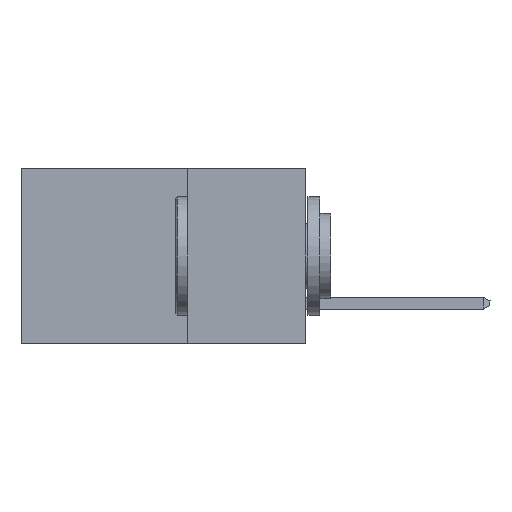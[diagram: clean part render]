
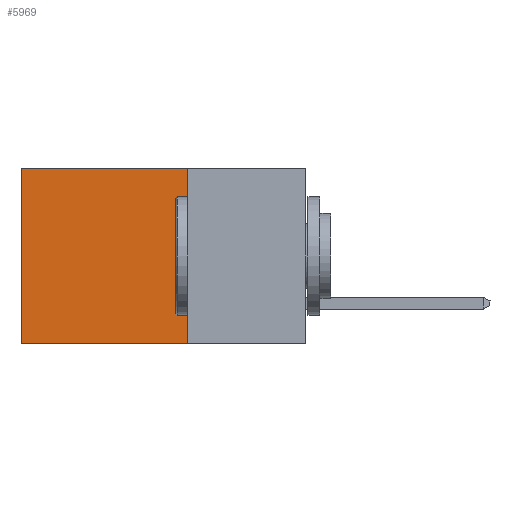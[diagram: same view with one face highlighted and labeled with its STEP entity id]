
A CAD part, left-side view. The second image highlights one B-rep face of the part: STEP entity #5969.
In plain terms, the highlighted planar face has unit normal (-1, 0, 0).
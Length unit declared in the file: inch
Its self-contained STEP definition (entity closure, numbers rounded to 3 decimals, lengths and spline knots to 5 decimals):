
#207 = VECTOR ( 'NONE', #5321, 39.37008 ) ;
#509 = EDGE_CURVE ( 'NONE', #4451, #18247, #7061, .T. ) ;
#1037 = VERTEX_POINT ( 'NONE', #16561 ) ;
#1584 = DIRECTION ( 'NONE',  ( 1., 0., 0. ) ) ;
#1895 = ORIENTED_EDGE ( 'NONE', *, *, #2058, .F. ) ;
#2058 = EDGE_CURVE ( 'NONE', #18247, #3424, #7263, .T. ) ;
#2236 = EDGE_CURVE ( 'NONE', #4451, #1037, #17257, .T. ) ;
#2767 = CARTESIAN_POINT ( 'NONE',  ( 0.298, 0.25, -0.37 ) ) ;
#2839 = VECTOR ( 'NONE', #12417, 39.37008 ) ;
#3405 = EDGE_LOOP ( 'NONE', ( #4843, #1895, #19400, #10245 ) ) ;
#3424 = VERTEX_POINT ( 'NONE', #19030 ) ;
#4451 = VERTEX_POINT ( 'NONE', #9928 ) ;
#4843 = ORIENTED_EDGE ( 'NONE', *, *, #10062, .T. ) ;
#5302 = VECTOR ( 'NONE', #11114, 39.37008 ) ;
#5321 = DIRECTION ( 'NONE',  ( 0., 0., -1. ) ) ;
#5491 = VECTOR ( 'NONE', #7530, 39.37008 ) ;
#5969 = ADVANCED_FACE ( 'NONE', ( #6856 ), #20221, .F. ) ;
#6165 = CARTESIAN_POINT ( 'NONE',  ( 0.298, 0.6, 0. ) ) ;
#6235 = CARTESIAN_POINT ( 'NONE',  ( 0.298, 0.25, 0. ) ) ;
#6415 = CARTESIAN_POINT ( 'NONE',  ( 0.298, 0.25, 0. ) ) ;
#6856 = FACE_OUTER_BOUND ( 'NONE', #3405, .T. ) ;
#7061 = LINE ( 'NONE', #14337, #207 ) ;
#7263 = LINE ( 'NONE', #2767, #2839 ) ;
#7530 = DIRECTION ( 'NONE',  ( 0., 0., -1. ) ) ;
#7910 = AXIS2_PLACEMENT_3D ( 'NONE', #6235, #1584, #14242 ) ;
#9928 = CARTESIAN_POINT ( 'NONE',  ( 0.298, 0.25, 0. ) ) ;
#10062 = EDGE_CURVE ( 'NONE', #1037, #3424, #15782, .T. ) ;
#10245 = ORIENTED_EDGE ( 'NONE', *, *, #2236, .T. ) ;
#11114 = DIRECTION ( 'NONE',  ( 0., 1., 0. ) ) ;
#12417 = DIRECTION ( 'NONE',  ( 0., 1., 0. ) ) ;
#14242 = DIRECTION ( 'NONE',  ( 0., 0., -1. ) ) ;
#14337 = CARTESIAN_POINT ( 'NONE',  ( 0.298, 0.25, 0. ) ) ;
#15782 = LINE ( 'NONE', #6165, #5491 ) ;
#16561 = CARTESIAN_POINT ( 'NONE',  ( 0.298, 0.6, 0. ) ) ;
#17257 = LINE ( 'NONE', #6415, #5302 ) ;
#17874 = CARTESIAN_POINT ( 'NONE',  ( 0.298, 0.25, -0.37 ) ) ;
#18247 = VERTEX_POINT ( 'NONE', #17874 ) ;
#19030 = CARTESIAN_POINT ( 'NONE',  ( 0.298, 0.6, -0.37 ) ) ;
#19400 = ORIENTED_EDGE ( 'NONE', *, *, #509, .F. ) ;
#20221 = PLANE ( 'NONE',  #7910 ) ;
